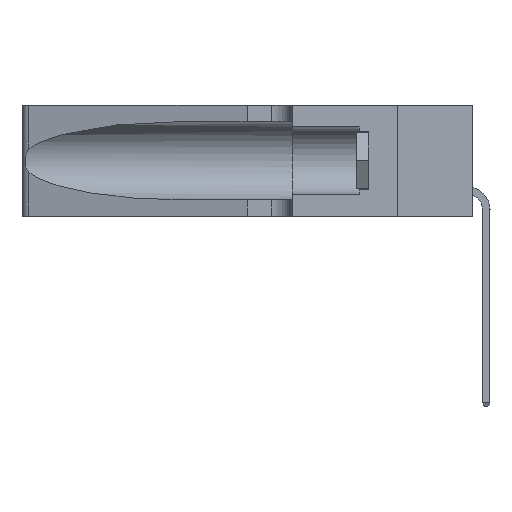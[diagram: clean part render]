
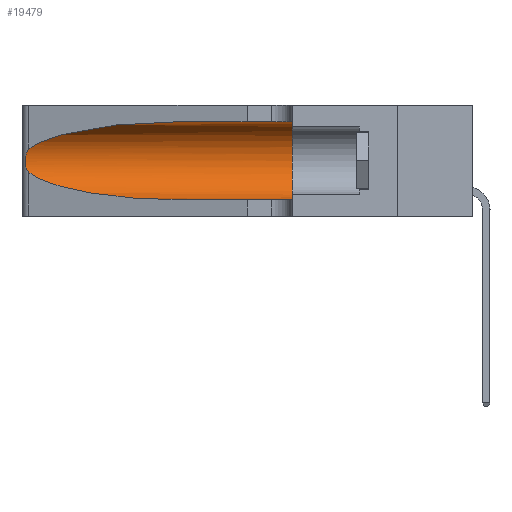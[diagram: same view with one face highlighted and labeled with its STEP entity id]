
A CAD part, left-side view. The second image highlights one B-rep face of the part: STEP entity #19479.
In plain terms, the highlighted cylindrical face has radius 3.308 mm (diameter 6.617 mm), a partial arc.
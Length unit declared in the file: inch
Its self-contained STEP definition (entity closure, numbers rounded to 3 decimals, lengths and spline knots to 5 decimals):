
#257 = CARTESIAN_POINT ( 'NONE',  ( 0.25854, 1.2359, 0.20912 ) ) ;
#621 = EDGE_CURVE ( 'NONE', #23595, #3800, #6494, .T. ) ;
#693 = CARTESIAN_POINT ( 'NONE',  ( 0.25639, 1.23186, 0.15144 ) ) ;
#1127 = ORIENTED_EDGE ( 'NONE', *, *, #621, .T. ) ;
#1627 = CARTESIAN_POINT ( 'NONE',  ( 0.1305, 1.61858, 0.185 ) ) ;
#1968 =( BOUNDED_CURVE ( )  B_SPLINE_CURVE ( 3, ( #2917, #8681, #4734, #14641 ),
 .UNSPECIFIED., .F., .F. ) 
 B_SPLINE_CURVE_WITH_KNOTS ( ( 4, 4 ),
 ( 1.5708, 2.84003 ),
 .UNSPECIFIED. ) 
 CURVE ( )  GEOMETRIC_REPRESENTATION_ITEM ( )  RATIONAL_B_SPLINE_CURVE ( ( 1., 0.87, 0.87, 1. ) ) 
 REPRESENTATION_ITEM ( '' )  );
#2917 = CARTESIAN_POINT ( 'NONE',  ( 0.1305, 0.72297, 0.31525 ) ) ;
#3094 = CARTESIAN_POINT ( 'NONE',  ( 0.1305, 1.61858, 0.31525 ) ) ;
#3166 = ORIENTED_EDGE ( 'NONE', *, *, #7310, .F. ) ;
#3438 = DIRECTION ( 'NONE',  ( 0., 0., 1. ) ) ;
#3800 = VERTEX_POINT ( 'NONE', #10400 ) ;
#3978 = CARTESIAN_POINT ( 'NONE',  ( 0.1305, 0.72297, 0.05475 ) ) ;
#4391 = CARTESIAN_POINT ( 'NONE',  ( 0.26075, 1.23896, 0.19203 ) ) ;
#4507 = LINE ( 'NONE', #3094, #17971 ) ;
#4691 = EDGE_CURVE ( 'NONE', #12349, #14942, #14318, .T. ) ;
#4734 = CARTESIAN_POINT ( 'NONE',  ( 0.2373, 1.15595, 0.28018 ) ) ;
#4864 = CARTESIAN_POINT ( 'NONE',  ( 0.25487, 1.22718, 0.14631 ) ) ;
#5015 = ORIENTED_EDGE ( 'NONE', *, *, #12769, .T. ) ;
#5728 = CARTESIAN_POINT ( 'NONE',  ( 0.1305, 1.61858, 0.05475 ) ) ;
#6216 = EDGE_CURVE ( 'NONE', #18460, #3800, #10535, .T. ) ;
#6392 = CARTESIAN_POINT ( 'NONE',  ( 0.25555, 1.22993, 0.14849 ) ) ;
#6494 = LINE ( 'NONE', #5728, #17789 ) ;
#6556 = CARTESIAN_POINT ( 'NONE',  ( 0.25487, 1.22718, 0.22369 ) ) ;
#7310 = EDGE_CURVE ( 'NONE', #20621, #18460, #4507, .T. ) ;
#7354 = ORIENTED_EDGE ( 'NONE', *, *, #6216, .F. ) ;
#7726 = CARTESIAN_POINT ( 'NONE',  ( 0.18966, 0.96281, 0.05475 ) ) ;
#8411 = CARTESIAN_POINT ( 'NONE',  ( 0.25487, 1.22718, 0.14631 ) ) ;
#8681 = CARTESIAN_POINT ( 'NONE',  ( 0.18966, 0.96281, 0.31525 ) ) ;
#8766 = CARTESIAN_POINT ( 'NONE',  ( 0.25789, 1.23486, 0.15765 ) ) ;
#9503 = CARTESIAN_POINT ( 'NONE',  ( 0.25487, 1.22718, 0.14631 ) ) ;
#9675 = CARTESIAN_POINT ( 'NONE',  ( 0.2373, 1.15595, 0.08982 ) ) ;
#10194 = CARTESIAN_POINT ( 'NONE',  ( 0.25487, 1.22718, 0.22369 ) ) ;
#10277 = CARTESIAN_POINT ( 'NONE',  ( 0.25639, 1.23184, 0.21858 ) ) ;
#10362 = CARTESIAN_POINT ( 'NONE',  ( 0.26075, 1.23896, 0.178 ) ) ;
#10366 = AXIS2_PLACEMENT_3D ( 'NONE', #15581, #21358, #3438 ) ;
#10400 = CARTESIAN_POINT ( 'NONE',  ( 0.1305, 0.35, 0.05475 ) ) ;
#10535 = CIRCLE ( 'NONE', #10366, 0.13025 ) ;
#11008 = CARTESIAN_POINT ( 'NONE',  ( 0.1305, 0.35, 0.31525 ) ) ;
#11299 =( BOUNDED_CURVE ( )  B_SPLINE_CURVE ( 3, ( #9503, #9675, #7726, #3978 ),
 .UNSPECIFIED., .F., .F. ) 
 B_SPLINE_CURVE_WITH_KNOTS ( ( 4, 4 ),
 ( 3.44316, 4.71239 ),
 .UNSPECIFIED. ) 
 CURVE ( )  GEOMETRIC_REPRESENTATION_ITEM ( )  RATIONAL_B_SPLINE_CURVE ( ( 1., 0.87, 0.87, 1. ) ) 
 REPRESENTATION_ITEM ( '' )  );
#11864 = DIRECTION ( 'NONE',  ( 0., -1., 0. ) ) ;
#12349 = VERTEX_POINT ( 'NONE', #6556 ) ;
#12706 = CARTESIAN_POINT ( 'NONE',  ( 0.26017, 1.23833, 0.17102 ) ) ;
#12769 = EDGE_CURVE ( 'NONE', #20621, #12349, #1968, .T. ) ;
#13080 = ORIENTED_EDGE ( 'NONE', *, *, #16205, .T. ) ;
#13459 = CARTESIAN_POINT ( 'NONE',  ( 0.1305, 0.72297, 0.05475 ) ) ;
#13933 = CARTESIAN_POINT ( 'NONE',  ( 0.25787, 1.23484, 0.2124 ) ) ;
#14318 = B_SPLINE_CURVE_WITH_KNOTS ( 'NONE', 3,
 ( #10194, #22197, #10277, #13933, #257, #20302, #4391, #10362, #12706, #18568, #8766, #693, #6392, #8411 ),
 .UNSPECIFIED., .F., .F.,
 ( 4, 2, 2, 2, 2, 2, 4 ),
 ( 0., 0.00027, 0.00053, 0.00107, 0.0016, 0.00187, 0.00214 ),
 .UNSPECIFIED. ) ;
#14641 = CARTESIAN_POINT ( 'NONE',  ( 0.25487, 1.22718, 0.22369 ) ) ;
#14942 = VERTEX_POINT ( 'NONE', #4864 ) ;
#14981 = EDGE_LOOP ( 'NONE', ( #5015, #19153, #13080, #1127, #7354, #3166 ) ) ;
#15581 = CARTESIAN_POINT ( 'NONE',  ( 0.1305, 0.35, 0.185 ) ) ;
#16205 = EDGE_CURVE ( 'NONE', #14942, #23595, #11299, .T. ) ;
#16242 = CARTESIAN_POINT ( 'NONE',  ( 0.1305, 0.72297, 0.31525 ) ) ;
#16912 = DIRECTION ( 'NONE',  ( 0., -1., 0. ) ) ;
#17383 = DIRECTION ( 'NONE',  ( 0., -1., 0. ) ) ;
#17464 = DIRECTION ( 'NONE',  ( 0., 0., -1. ) ) ;
#17789 = VECTOR ( 'NONE', #11864, 39.37008 ) ;
#17935 = CYLINDRICAL_SURFACE ( 'NONE', #22845, 0.13025 ) ;
#17971 = VECTOR ( 'NONE', #16912, 39.37008 ) ;
#18460 = VERTEX_POINT ( 'NONE', #11008 ) ;
#18562 = FACE_OUTER_BOUND ( 'NONE', #14981, .T. ) ;
#18568 = CARTESIAN_POINT ( 'NONE',  ( 0.25856, 1.23593, 0.16098 ) ) ;
#19153 = ORIENTED_EDGE ( 'NONE', *, *, #4691, .T. ) ;
#19479 = ADVANCED_FACE ( 'NONE', ( #18562 ), #17935, .F. ) ;
#20302 = CARTESIAN_POINT ( 'NONE',  ( 0.26018, 1.23835, 0.19895 ) ) ;
#20621 = VERTEX_POINT ( 'NONE', #16242 ) ;
#21358 = DIRECTION ( 'NONE',  ( 0., 1., 0. ) ) ;
#22197 = CARTESIAN_POINT ( 'NONE',  ( 0.25555, 1.22994, 0.2215 ) ) ;
#22845 = AXIS2_PLACEMENT_3D ( 'NONE', #1627, #17383, #17464 ) ;
#23595 = VERTEX_POINT ( 'NONE', #13459 ) ;
